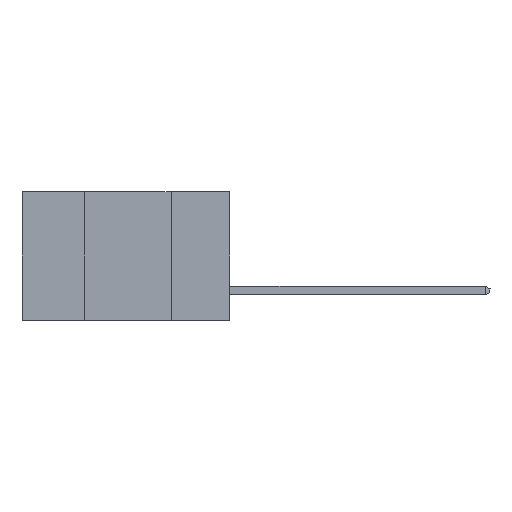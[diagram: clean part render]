
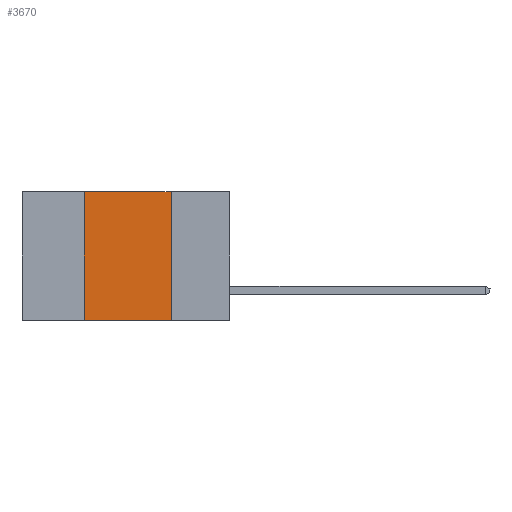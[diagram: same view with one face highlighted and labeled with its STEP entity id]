
A CAD part, left-side view. The second image highlights one B-rep face of the part: STEP entity #3670.
In plain terms, the highlighted planar face has unit normal (-1, 0, 0).
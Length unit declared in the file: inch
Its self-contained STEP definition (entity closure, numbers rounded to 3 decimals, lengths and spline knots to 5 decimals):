
#200 = AXIS2_PLACEMENT_3D ( 'NONE', #5871, #6742, #10262 ) ;
#230 = ORIENTED_EDGE ( 'NONE', *, *, #2939, .F. ) ;
#278 = ORIENTED_EDGE ( 'NONE', *, *, #1419, .F. ) ;
#382 = VECTOR ( 'NONE', #7874, 39.37008 ) ;
#427 = CARTESIAN_POINT ( 'NONE',  ( 0., 0.42, -0.37 ) ) ;
#642 = PLANE ( 'NONE',  #200 ) ;
#682 = CARTESIAN_POINT ( 'NONE',  ( 0., 0.17, -0.37 ) ) ;
#1419 = EDGE_CURVE ( 'NONE', #2369, #4201, #4810, .T. ) ;
#2369 = VERTEX_POINT ( 'NONE', #8305 ) ;
#2422 = VERTEX_POINT ( 'NONE', #682 ) ;
#2618 = ORIENTED_EDGE ( 'NONE', *, *, #4116, .T. ) ;
#2745 = VECTOR ( 'NONE', #6091, 39.37008 ) ;
#2939 = EDGE_CURVE ( 'NONE', #4201, #5187, #10588, .T. ) ;
#3232 = FACE_OUTER_BOUND ( 'NONE', #9070, .T. ) ;
#3670 = ADVANCED_FACE ( 'NONE', ( #3232 ), #642, .F. ) ;
#4116 = EDGE_CURVE ( 'NONE', #2369, #2422, #9635, .T. ) ;
#4201 = VERTEX_POINT ( 'NONE', #8282 ) ;
#4757 = DIRECTION ( 'NONE',  ( 0., 0., 1. ) ) ;
#4810 = LINE ( 'NONE', #427, #11132 ) ;
#5187 = VERTEX_POINT ( 'NONE', #11013 ) ;
#5205 = EDGE_CURVE ( 'NONE', #5187, #2422, #10897, .T. ) ;
#5871 = CARTESIAN_POINT ( 'NONE',  ( 0., 0.6, 0. ) ) ;
#6091 = DIRECTION ( 'NONE',  ( 0., -1., 0. ) ) ;
#6135 = CARTESIAN_POINT ( 'NONE',  ( 0., 0.6, 0. ) ) ;
#6152 = CARTESIAN_POINT ( 'NONE',  ( 0., 0.6, -0.37 ) ) ;
#6396 = CARTESIAN_POINT ( 'NONE',  ( 0., 0.17, -0.37 ) ) ;
#6401 = ORIENTED_EDGE ( 'NONE', *, *, #5205, .F. ) ;
#6742 = DIRECTION ( 'NONE',  ( 1., 0., 0. ) ) ;
#7874 = DIRECTION ( 'NONE',  ( 0., -1., 0. ) ) ;
#7941 = VECTOR ( 'NONE', #8258, 39.37008 ) ;
#8258 = DIRECTION ( 'NONE',  ( 0., 0., -1. ) ) ;
#8282 = CARTESIAN_POINT ( 'NONE',  ( 0., 0.42, 0. ) ) ;
#8305 = CARTESIAN_POINT ( 'NONE',  ( 0., 0.42, -0.37 ) ) ;
#9070 = EDGE_LOOP ( 'NONE', ( #6401, #230, #278, #2618 ) ) ;
#9635 = LINE ( 'NONE', #6152, #2745 ) ;
#10262 = DIRECTION ( 'NONE',  ( 0., 0., -1. ) ) ;
#10588 = LINE ( 'NONE', #6135, #382 ) ;
#10897 = LINE ( 'NONE', #6396, #7941 ) ;
#11013 = CARTESIAN_POINT ( 'NONE',  ( 0., 0.17, 0. ) ) ;
#11132 = VECTOR ( 'NONE', #4757, 39.37008 ) ;
